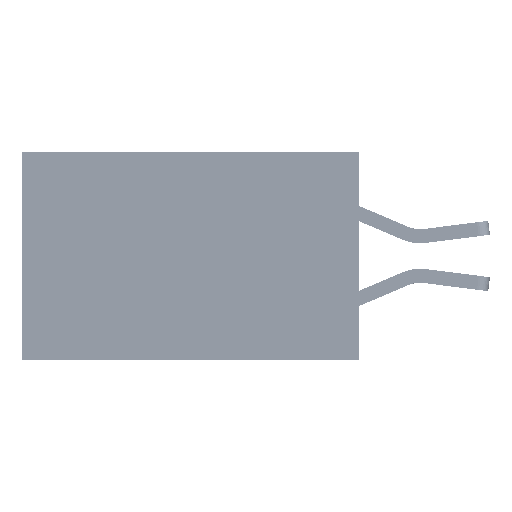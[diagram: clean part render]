
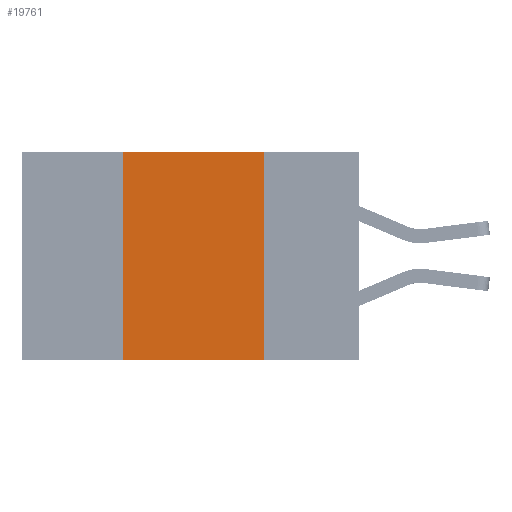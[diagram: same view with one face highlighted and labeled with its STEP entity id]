
A CAD part, left-side view. The second image highlights one B-rep face of the part: STEP entity #19761.
In plain terms, the highlighted planar face has unit normal (-1, 0, 0).
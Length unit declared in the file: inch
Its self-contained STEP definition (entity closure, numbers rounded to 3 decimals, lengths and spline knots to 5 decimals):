
#232 = DIRECTION ( 'NONE',  ( 0., 0., 1. ) ) ;
#418 = CARTESIAN_POINT ( 'NONE',  ( 0., 0.6, -0.37 ) ) ;
#3649 = DIRECTION ( 'NONE',  ( 1., 0., 0. ) ) ;
#4184 = VECTOR ( 'NONE', #38510, 39.37008 ) ;
#4552 = LINE ( 'NONE', #32307, #21761 ) ;
#5175 = EDGE_CURVE ( 'NONE', #15837, #41339, #15316, .T. ) ;
#6963 = DIRECTION ( 'NONE',  ( 0., -1., 0. ) ) ;
#8926 = VECTOR ( 'NONE', #232, 39.37008 ) ;
#9698 = FACE_OUTER_BOUND ( 'NONE', #15244, .T. ) ;
#9797 = DIRECTION ( 'NONE',  ( 0., 0., -1. ) ) ;
#10566 = CARTESIAN_POINT ( 'NONE',  ( 0., 0.42, 0. ) ) ;
#13194 = CARTESIAN_POINT ( 'NONE',  ( 0., 0.42, 0. ) ) ;
#15244 = EDGE_LOOP ( 'NONE', ( #32030, #29996, #38665, #31985 ) ) ;
#15316 = LINE ( 'NONE', #418, #38901 ) ;
#15837 = VERTEX_POINT ( 'NONE', #34415 ) ;
#16091 = EDGE_CURVE ( 'NONE', #15837, #40537, #17559, .T. ) ;
#17559 = LINE ( 'NONE', #13194, #8926 ) ;
#17608 = CARTESIAN_POINT ( 'NONE',  ( 0., 0.17, -0.37 ) ) ;
#19761 = ADVANCED_FACE ( 'NONE', ( #9698 ), #23035, .F. ) ;
#19837 = CARTESIAN_POINT ( 'NONE',  ( 0., 0.6, 0. ) ) ;
#19924 = CARTESIAN_POINT ( 'NONE',  ( 0., 0.17, 0. ) ) ;
#21761 = VECTOR ( 'NONE', #9797, 39.37008 ) ;
#23035 = PLANE ( 'NONE',  #41672 ) ;
#24681 = EDGE_CURVE ( 'NONE', #37026, #41339, #4552, .T. ) ;
#26270 = DIRECTION ( 'NONE',  ( 0., 0., -1. ) ) ;
#28808 = CARTESIAN_POINT ( 'NONE',  ( 0., 0.6, 0. ) ) ;
#29311 = EDGE_CURVE ( 'NONE', #40537, #37026, #29953, .T. ) ;
#29953 = LINE ( 'NONE', #28808, #4184 ) ;
#29996 = ORIENTED_EDGE ( 'NONE', *, *, #29311, .F. ) ;
#31985 = ORIENTED_EDGE ( 'NONE', *, *, #5175, .T. ) ;
#32030 = ORIENTED_EDGE ( 'NONE', *, *, #24681, .F. ) ;
#32307 = CARTESIAN_POINT ( 'NONE',  ( 0., 0.17, 0. ) ) ;
#34415 = CARTESIAN_POINT ( 'NONE',  ( 0., 0.42, -0.37 ) ) ;
#37026 = VERTEX_POINT ( 'NONE', #19924 ) ;
#38510 = DIRECTION ( 'NONE',  ( 0., -1., 0. ) ) ;
#38665 = ORIENTED_EDGE ( 'NONE', *, *, #16091, .F. ) ;
#38901 = VECTOR ( 'NONE', #6963, 39.37008 ) ;
#40537 = VERTEX_POINT ( 'NONE', #10566 ) ;
#41339 = VERTEX_POINT ( 'NONE', #17608 ) ;
#41672 = AXIS2_PLACEMENT_3D ( 'NONE', #19837, #3649, #26270 ) ;
